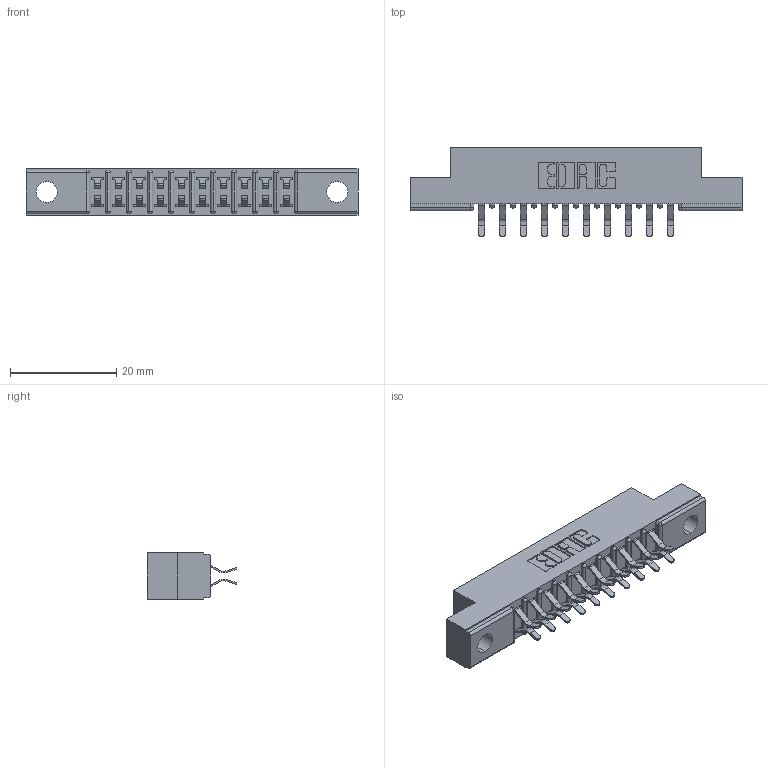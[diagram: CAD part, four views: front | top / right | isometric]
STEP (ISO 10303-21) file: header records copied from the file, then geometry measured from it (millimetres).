
FILE_DESCRIPTION (( 'STEP AP203' ), '1' );
FILE_NAME ('357-020-456-204.STEP', '2020-10-02T22:19:48', ( '' ), ( '' ), 'SwSTEP 2.0', 'SolidWorks 2020', '' );
FILE_SCHEMA (( 'CONFIG_CONTROL_DESIGN' ));
Length unit declared in the file: inch
Products named in the file (3): 307-290-001_556; 307 Part_.156 Dia Mounting Holes; 357-020-456-204
Assembly tree (21 placements, depth 2):
  357-020-456-204
    307 Part_.156 Dia Mounting Holes
    307-290-001_556  x20
Bounding box: 62.64 x 16.97 x 8.71 mm (x, y, z)
Volume: 3988.9 mm3; surface area: 6288 mm2
Topology: 21 solids, 21 shells, 1143 faces, 3199 edges, 2074 vertices
Faces by surface type: plane 744, cylinder 377, sphere 22
Entity records: 13360 total; most frequent: CARTESIAN_POINT 2200, ORIENTED_EDGE 2174, DIRECTION 2161, EDGE_CURVE 1087, LINE 827, VECTOR 827, VERTEX_POINT 706, AXIS2_PLACEMENT_3D 667
